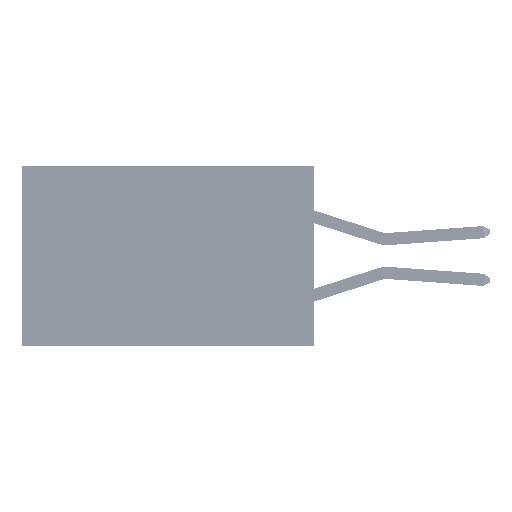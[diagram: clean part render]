
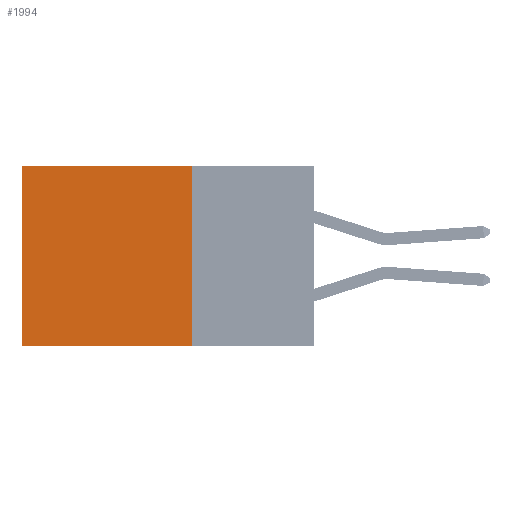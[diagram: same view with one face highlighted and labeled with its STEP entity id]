
A CAD part, left-side view. The second image highlights one B-rep face of the part: STEP entity #1994.
In plain terms, the highlighted planar face has unit normal (-1, 0, 0).
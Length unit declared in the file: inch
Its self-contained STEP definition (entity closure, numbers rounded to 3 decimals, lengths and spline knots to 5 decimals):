
#774 = DIRECTION ( 'NONE',  ( 0., 0., -1. ) ) ;
#1684 = CARTESIAN_POINT ( 'NONE',  ( 0.2875, 0.6, 0. ) ) ;
#1994 = ADVANCED_FACE ( 'NONE', ( #16199 ), #27359, .F. ) ;
#2409 = CARTESIAN_POINT ( 'NONE',  ( 0.2875, 0.6, 0. ) ) ;
#3777 = CARTESIAN_POINT ( 'NONE',  ( 0.2875, 0.25, 0. ) ) ;
#3931 = EDGE_CURVE ( 'NONE', #17793, #37776, #47440, .T. ) ;
#3953 = EDGE_CURVE ( 'NONE', #24146, #41413, #13141, .T. ) ;
#4454 = CARTESIAN_POINT ( 'NONE',  ( 0.2875, 0.6, -0.37 ) ) ;
#4802 = ORIENTED_EDGE ( 'NONE', *, *, #28220, .T. ) ;
#5525 = ORIENTED_EDGE ( 'NONE', *, *, #3953, .T. ) ;
#8395 = DIRECTION ( 'NONE',  ( 0., 1., 0. ) ) ;
#8506 = ORIENTED_EDGE ( 'NONE', *, *, #3931, .F. ) ;
#9784 = CARTESIAN_POINT ( 'NONE',  ( 0.2875, 0.25, 0. ) ) ;
#12998 = CARTESIAN_POINT ( 'NONE',  ( 0.2875, 0.25, -0.37 ) ) ;
#13141 = LINE ( 'NONE', #1684, #32453 ) ;
#15959 = DIRECTION ( 'NONE',  ( 1., 0., 0. ) ) ;
#16199 = FACE_OUTER_BOUND ( 'NONE', #22996, .T. ) ;
#16383 = CARTESIAN_POINT ( 'NONE',  ( 0.2875, 0.25, 0. ) ) ;
#17793 = VERTEX_POINT ( 'NONE', #9784 ) ;
#19757 = VECTOR ( 'NONE', #20844, 39.37008 ) ;
#20430 = DIRECTION ( 'NONE',  ( 0., 1., 0. ) ) ;
#20844 = DIRECTION ( 'NONE',  ( 0., 0., -1. ) ) ;
#22894 = AXIS2_PLACEMENT_3D ( 'NONE', #3777, #15959, #774 ) ;
#22925 = VECTOR ( 'NONE', #20430, 39.37008 ) ;
#22996 = EDGE_LOOP ( 'NONE', ( #5525, #24548, #8506, #4802 ) ) ;
#23663 = LINE ( 'NONE', #12998, #22925 ) ;
#24146 = VERTEX_POINT ( 'NONE', #2409 ) ;
#24548 = ORIENTED_EDGE ( 'NONE', *, *, #31397, .F. ) ;
#26313 = CARTESIAN_POINT ( 'NONE',  ( 0.2875, 0.25, -0.37 ) ) ;
#27285 = LINE ( 'NONE', #42459, #30761 ) ;
#27359 = PLANE ( 'NONE',  #22894 ) ;
#28220 = EDGE_CURVE ( 'NONE', #17793, #24146, #27285, .T. ) ;
#30761 = VECTOR ( 'NONE', #8395, 39.37008 ) ;
#31397 = EDGE_CURVE ( 'NONE', #37776, #41413, #23663, .T. ) ;
#32453 = VECTOR ( 'NONE', #35985, 39.37008 ) ;
#35985 = DIRECTION ( 'NONE',  ( 0., 0., -1. ) ) ;
#37776 = VERTEX_POINT ( 'NONE', #26313 ) ;
#41413 = VERTEX_POINT ( 'NONE', #4454 ) ;
#42459 = CARTESIAN_POINT ( 'NONE',  ( 0.2875, 0.25, 0. ) ) ;
#47440 = LINE ( 'NONE', #16383, #19757 ) ;
